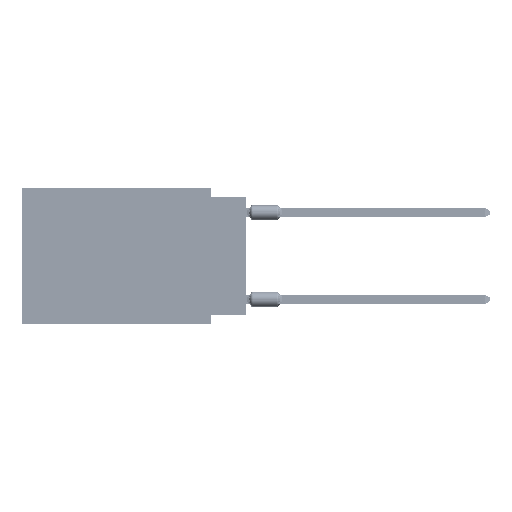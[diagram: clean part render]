
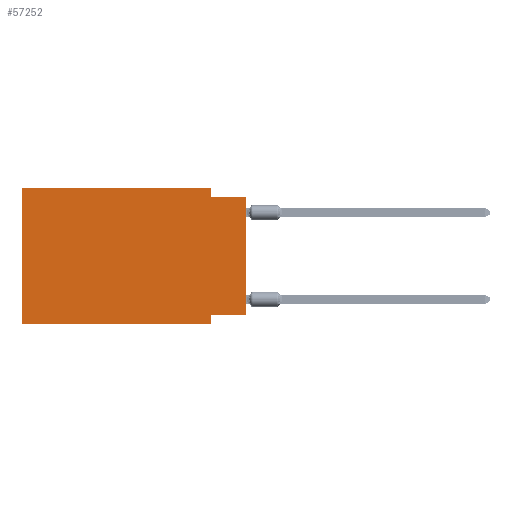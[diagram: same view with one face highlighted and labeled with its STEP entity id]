
A CAD part, left-side view. The second image highlights one B-rep face of the part: STEP entity #57252.
In plain terms, the highlighted planar face has unit normal (-1, 0, 0).
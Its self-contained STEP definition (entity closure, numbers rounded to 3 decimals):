
#2389 = CARTESIAN_POINT ( 'NONE',  ( 0., 0., -0.635 ) ) ;
#2501 = LINE ( 'NONE', #24208, #17014 ) ;
#4690 = ORIENTED_EDGE ( 'NONE', *, *, #59505, .F. ) ;
#8546 = ORIENTED_EDGE ( 'NONE', *, *, #10623, .F. ) ;
#10623 = EDGE_CURVE ( 'NONE', #57345, #32160, #2501, .T. ) ;
#11953 = VERTEX_POINT ( 'NONE', #62960 ) ;
#12025 = EDGE_CURVE ( 'NONE', #47210, #66935, #69377, .T. ) ;
#12040 = CARTESIAN_POINT ( 'NONE',  ( 0., 16.383, 0. ) ) ;
#12734 = LINE ( 'NONE', #12040, #51921 ) ;
#13275 = ORIENTED_EDGE ( 'NONE', *, *, #12025, .T. ) ;
#14771 = ORIENTED_EDGE ( 'NONE', *, *, #27771, .F. ) ;
#15031 = DIRECTION ( 'NONE',  ( 0., 0., -1. ) ) ;
#15402 = VERTEX_POINT ( 'NONE', #52586 ) ;
#15724 = PLANE ( 'NONE',  #31386 ) ;
#16698 = LINE ( 'NONE', #55532, #45590 ) ;
#17014 = VECTOR ( 'NONE', #45958, 1000. ) ;
#18434 = VECTOR ( 'NONE', #68701, 1000. ) ;
#21357 = EDGE_CURVE ( 'NONE', #52131, #52654, #40217, .T. ) ;
#23278 = LINE ( 'NONE', #33633, #29999 ) ;
#23349 = CARTESIAN_POINT ( 'NONE',  ( 0., 2.54, -0.635 ) ) ;
#24164 = CARTESIAN_POINT ( 'NONE',  ( 0., 16.383, 0. ) ) ;
#24208 = CARTESIAN_POINT ( 'NONE',  ( 0., 2.54, 0. ) ) ;
#24516 = CARTESIAN_POINT ( 'NONE',  ( 0., 16.383, 0. ) ) ;
#26550 = DIRECTION ( 'NONE',  ( 0., 0., 1. ) ) ;
#27771 = EDGE_CURVE ( 'NONE', #47210, #15402, #16698, .T. ) ;
#28421 = DIRECTION ( 'NONE',  ( 0., 1., 0. ) ) ;
#29999 = VECTOR ( 'NONE', #66797, 1000. ) ;
#30203 = DIRECTION ( 'NONE',  ( 0., 0., -1. ) ) ;
#31386 = AXIS2_PLACEMENT_3D ( 'NONE', #41763, #59216, #15031 ) ;
#32160 = VERTEX_POINT ( 'NONE', #23349 ) ;
#33206 = CARTESIAN_POINT ( 'NONE',  ( 0., 16.383, -9.906 ) ) ;
#33633 = CARTESIAN_POINT ( 'NONE',  ( 0., 16.383, -9.906 ) ) ;
#33747 = EDGE_CURVE ( 'NONE', #52131, #11953, #23278, .T. ) ;
#33883 = CARTESIAN_POINT ( 'NONE',  ( 0., 2.54, -9.906 ) ) ;
#35888 = CARTESIAN_POINT ( 'NONE',  ( 0., 0., -9.271 ) ) ;
#40217 = LINE ( 'NONE', #24164, #46278 ) ;
#41243 = LINE ( 'NONE', #52293, #18434 ) ;
#41763 = CARTESIAN_POINT ( 'NONE',  ( 0., 16.383, 0. ) ) ;
#43210 = EDGE_CURVE ( 'NONE', #15402, #11953, #66348, .T. ) ;
#43515 = CARTESIAN_POINT ( 'NONE',  ( 0., 2.54, 0. ) ) ;
#45536 = ORIENTED_EDGE ( 'NONE', *, *, #47206, .F. ) ;
#45590 = VECTOR ( 'NONE', #28421, 1000. ) ;
#45958 = DIRECTION ( 'NONE',  ( 0., 0., -1. ) ) ;
#46278 = VECTOR ( 'NONE', #61278, 1000. ) ;
#46683 = VECTOR ( 'NONE', #30203, 1000. ) ;
#47206 = EDGE_CURVE ( 'NONE', #32160, #66935, #41243, .T. ) ;
#47210 = VERTEX_POINT ( 'NONE', #35888 ) ;
#49220 = ORIENTED_EDGE ( 'NONE', *, *, #33747, .T. ) ;
#49627 = ORIENTED_EDGE ( 'NONE', *, *, #43210, .F. ) ;
#50161 = DIRECTION ( 'NONE',  ( 0., -1., 0. ) ) ;
#51921 = VECTOR ( 'NONE', #50161, 1000. ) ;
#52131 = VERTEX_POINT ( 'NONE', #33206 ) ;
#52293 = CARTESIAN_POINT ( 'NONE',  ( 0., 0., -0.635 ) ) ;
#52382 = VECTOR ( 'NONE', #26550, 1000. ) ;
#52586 = CARTESIAN_POINT ( 'NONE',  ( 0., 2.54, -9.271 ) ) ;
#52654 = VERTEX_POINT ( 'NONE', #24516 ) ;
#54015 = CARTESIAN_POINT ( 'NONE',  ( 0., 0., 0. ) ) ;
#55532 = CARTESIAN_POINT ( 'NONE',  ( 0., 0., -9.271 ) ) ;
#57252 = ADVANCED_FACE ( 'NONE', ( #63871 ), #15724, .F. ) ;
#57345 = VERTEX_POINT ( 'NONE', #43515 ) ;
#58318 = EDGE_LOOP ( 'NONE', ( #13275, #45536, #8546, #4690, #69735, #49220, #49627, #14771 ) ) ;
#59216 = DIRECTION ( 'NONE',  ( 1., 0., 0. ) ) ;
#59505 = EDGE_CURVE ( 'NONE', #52654, #57345, #12734, .T. ) ;
#61278 = DIRECTION ( 'NONE',  ( 0., 0., 1. ) ) ;
#62960 = CARTESIAN_POINT ( 'NONE',  ( 0., 2.54, -9.906 ) ) ;
#63871 = FACE_OUTER_BOUND ( 'NONE', #58318, .T. ) ;
#66348 = LINE ( 'NONE', #33883, #46683 ) ;
#66797 = DIRECTION ( 'NONE',  ( 0., -1., 0. ) ) ;
#66935 = VERTEX_POINT ( 'NONE', #2389 ) ;
#68701 = DIRECTION ( 'NONE',  ( 0., -1., 0. ) ) ;
#69377 = LINE ( 'NONE', #54015, #52382 ) ;
#69735 = ORIENTED_EDGE ( 'NONE', *, *, #21357, .F. ) ;
